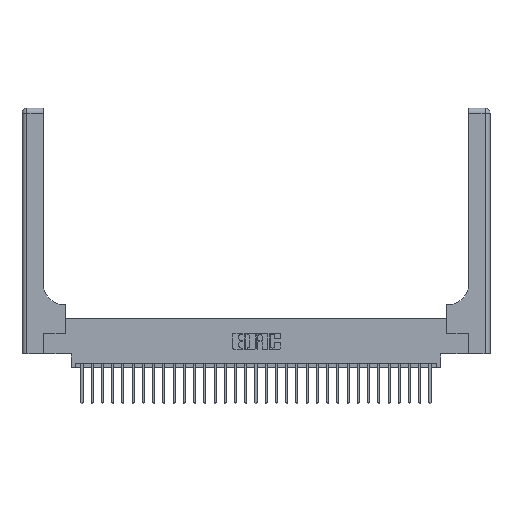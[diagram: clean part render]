
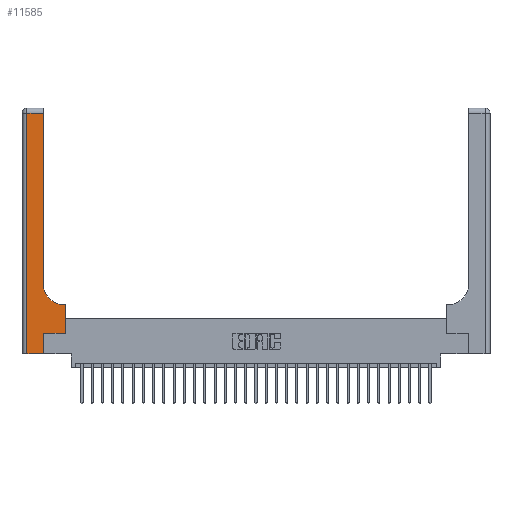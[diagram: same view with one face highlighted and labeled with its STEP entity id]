
A CAD part, top view. The second image highlights one B-rep face of the part: STEP entity #11585.
In plain terms, the highlighted planar face has unit normal (0, 0, 1).
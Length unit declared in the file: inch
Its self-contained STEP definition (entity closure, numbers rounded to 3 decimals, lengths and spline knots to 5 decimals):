
#195 = ORIENTED_EDGE ( 'NONE', *, *, #5107, .T. ) ;
#230 = DIRECTION ( 'NONE',  ( -1., 0., 0. ) ) ;
#773 = VERTEX_POINT ( 'NONE', #4619 ) ;
#1105 = DIRECTION ( 'NONE',  ( -1., 0., 0. ) ) ;
#1269 = CARTESIAN_POINT ( 'NONE',  ( 0.06, 2.94, 0.37 ) ) ;
#2321 = EDGE_CURVE ( 'NONE', #13867, #16828, #17605, .T. ) ;
#2589 = EDGE_CURVE ( 'NONE', #16691, #13867, #23856, .T. ) ;
#2597 = DIRECTION ( 'NONE',  ( 0., -1., 0. ) ) ;
#3067 = DIRECTION ( 'NONE',  ( 0., 1., 0. ) ) ;
#4061 = VERTEX_POINT ( 'NONE', #1269 ) ;
#4363 = DIRECTION ( 'NONE',  ( -1., 0., 0. ) ) ;
#4619 = CARTESIAN_POINT ( 'NONE',  ( 0.528, 0.6, 0.37 ) ) ;
#5107 = EDGE_CURVE ( 'NONE', #4061, #16691, #8192, .T. ) ;
#5283 = EDGE_CURVE ( 'NONE', #773, #22446, #27139, .T. ) ;
#5632 = CARTESIAN_POINT ( 'NONE',  ( 0.528, 0.25, 0.37 ) ) ;
#5882 = CARTESIAN_POINT ( 'NONE',  ( 0.26, 3., 0.37 ) ) ;
#6089 = VECTOR ( 'NONE', #11782, 39.37008 ) ;
#6113 = EDGE_CURVE ( 'NONE', #27909, #10127, #17336, .T. ) ;
#6294 = EDGE_LOOP ( 'NONE', ( #15407, #22066, #195, #18957, #15068, #15773, #11200, #23832, #18619 ) ) ;
#6575 = EDGE_CURVE ( 'NONE', #22446, #27909, #19410, .T. ) ;
#7520 = CARTESIAN_POINT ( 'NONE',  ( 0.265, 0., 0.37 ) ) ;
#7537 = DIRECTION ( 'NONE',  ( 0., 0., -1. ) ) ;
#7897 = DIRECTION ( 'NONE',  ( 0., 1., 0. ) ) ;
#8192 = LINE ( 'NONE', #11610, #18786 ) ;
#8539 = VECTOR ( 'NONE', #1105, 39.37008 ) ;
#10127 = VERTEX_POINT ( 'NONE', #16925 ) ;
#10130 = CARTESIAN_POINT ( 'NONE',  ( 0.51, 0.6, 0.37 ) ) ;
#10262 = CARTESIAN_POINT ( 'NONE',  ( 0.06, 0., 0.37 ) ) ;
#10839 = CARTESIAN_POINT ( 'NONE',  ( 0., 0., 0.37 ) ) ;
#11200 = ORIENTED_EDGE ( 'NONE', *, *, #27648, .T. ) ;
#11585 = ADVANCED_FACE ( 'NONE', ( #29114 ), #22176, .F. ) ;
#11610 = CARTESIAN_POINT ( 'NONE',  ( 0.06, 3., 0.37 ) ) ;
#11782 = DIRECTION ( 'NONE',  ( 1., 0., 0. ) ) ;
#13867 = VERTEX_POINT ( 'NONE', #7520 ) ;
#15068 = ORIENTED_EDGE ( 'NONE', *, *, #2321, .T. ) ;
#15407 = ORIENTED_EDGE ( 'NONE', *, *, #6113, .T. ) ;
#15610 = CARTESIAN_POINT ( 'NONE',  ( 0., 3., 0.37 ) ) ;
#15773 = ORIENTED_EDGE ( 'NONE', *, *, #26868, .T. ) ;
#15907 = VECTOR ( 'NONE', #7897, 39.37008 ) ;
#16249 = VERTEX_POINT ( 'NONE', #24111 ) ;
#16691 = VERTEX_POINT ( 'NONE', #10262 ) ;
#16828 = VERTEX_POINT ( 'NONE', #26337 ) ;
#16925 = CARTESIAN_POINT ( 'NONE',  ( 0.26, 2.94, 0.37 ) ) ;
#17248 = VECTOR ( 'NONE', #28772, 39.37008 ) ;
#17326 = VECTOR ( 'NONE', #230, 39.37008 ) ;
#17336 = LINE ( 'NONE', #5882, #23948 ) ;
#17605 = LINE ( 'NONE', #27712, #28760 ) ;
#17906 = DIRECTION ( 'NONE',  ( 0., 0., -1. ) ) ;
#18619 = ORIENTED_EDGE ( 'NONE', *, *, #6575, .T. ) ;
#18786 = VECTOR ( 'NONE', #2597, 39.37008 ) ;
#18957 = ORIENTED_EDGE ( 'NONE', *, *, #2589, .T. ) ;
#19410 = CIRCLE ( 'NONE', #24231, 0.25 ) ;
#20935 = AXIS2_PLACEMENT_3D ( 'NONE', #15610, #17906, #4363 ) ;
#21027 = CARTESIAN_POINT ( 'NONE',  ( 0.51, 0.85, 0.37 ) ) ;
#21422 = CARTESIAN_POINT ( 'NONE',  ( 0.26, 0.6, 0.37 ) ) ;
#21633 = DIRECTION ( 'NONE',  ( 0., 1., 0. ) ) ;
#22066 = ORIENTED_EDGE ( 'NONE', *, *, #28083, .T. ) ;
#22176 = PLANE ( 'NONE',  #20935 ) ;
#22446 = VERTEX_POINT ( 'NONE', #10130 ) ;
#23258 = DIRECTION ( 'NONE',  ( 1., 0., 0. ) ) ;
#23832 = ORIENTED_EDGE ( 'NONE', *, *, #5283, .T. ) ;
#23856 = LINE ( 'NONE', #10839, #17248 ) ;
#23948 = VECTOR ( 'NONE', #21633, 39.37008 ) ;
#24024 = LINE ( 'NONE', #27445, #6089 ) ;
#24111 = CARTESIAN_POINT ( 'NONE',  ( 0.528, 0.25, 0.37 ) ) ;
#24231 = AXIS2_PLACEMENT_3D ( 'NONE', #21027, #7537, #23258 ) ;
#26337 = CARTESIAN_POINT ( 'NONE',  ( 0.265, 0.25, 0.37 ) ) ;
#26868 = EDGE_CURVE ( 'NONE', #16828, #16249, #24024, .T. ) ;
#27139 = LINE ( 'NONE', #21422, #8539 ) ;
#27194 = CARTESIAN_POINT ( 'NONE',  ( 0., 2.94, 0.37 ) ) ;
#27445 = CARTESIAN_POINT ( 'NONE',  ( 0.265, 0.25, 0.37 ) ) ;
#27648 = EDGE_CURVE ( 'NONE', #16249, #773, #27806, .T. ) ;
#27712 = CARTESIAN_POINT ( 'NONE',  ( 0.265, 0., 0.37 ) ) ;
#27806 = LINE ( 'NONE', #5632, #15907 ) ;
#27909 = VERTEX_POINT ( 'NONE', #28776 ) ;
#28083 = EDGE_CURVE ( 'NONE', #10127, #4061, #28481, .T. ) ;
#28481 = LINE ( 'NONE', #27194, #17326 ) ;
#28760 = VECTOR ( 'NONE', #3067, 39.37008 ) ;
#28772 = DIRECTION ( 'NONE',  ( 1., 0., 0. ) ) ;
#28776 = CARTESIAN_POINT ( 'NONE',  ( 0.26, 0.85, 0.37 ) ) ;
#29114 = FACE_OUTER_BOUND ( 'NONE', #6294, .T. ) ;
